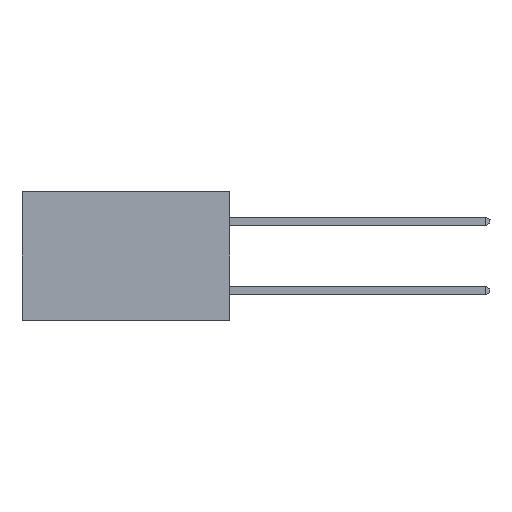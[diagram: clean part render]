
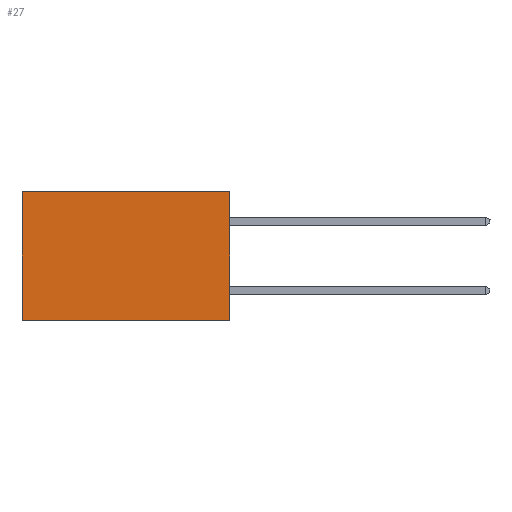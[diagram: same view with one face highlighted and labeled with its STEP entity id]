
A CAD part, left-side view. The second image highlights one B-rep face of the part: STEP entity #27.
In plain terms, the highlighted planar face has unit normal (-1, 0, 0).
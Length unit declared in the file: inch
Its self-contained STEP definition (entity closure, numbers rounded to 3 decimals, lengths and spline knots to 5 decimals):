
#27 = ADVANCED_FACE ( 'NONE', ( #2686 ), #23878, .F. ) ;
#100 = VECTOR ( 'NONE', #18522, 39.37008 ) ;
#650 = CARTESIAN_POINT ( 'NONE',  ( 0.298, 0.6, -0.37 ) ) ;
#1369 = LINE ( 'NONE', #11247, #26926 ) ;
#1914 = CARTESIAN_POINT ( 'NONE',  ( 0.298, 0.6, 0. ) ) ;
#2084 = LINE ( 'NONE', #24948, #100 ) ;
#2681 = CARTESIAN_POINT ( 'NONE',  ( 0.298, 0., 0. ) ) ;
#2686 = FACE_OUTER_BOUND ( 'NONE', #17113, .T. ) ;
#2839 = DIRECTION ( 'NONE',  ( 0., 0., -1. ) ) ;
#3073 = AXIS2_PLACEMENT_3D ( 'NONE', #2681, #17654, #5064 ) ;
#3188 = ORIENTED_EDGE ( 'NONE', *, *, #8913, .T. ) ;
#4081 = CARTESIAN_POINT ( 'NONE',  ( 0.298, 0., 0. ) ) ;
#4966 = ORIENTED_EDGE ( 'NONE', *, *, #25215, .F. ) ;
#5064 = DIRECTION ( 'NONE',  ( 0., 0., -1. ) ) ;
#8871 = VERTEX_POINT ( 'NONE', #17053 ) ;
#8913 = EDGE_CURVE ( 'NONE', #12993, #17207, #2084, .T. ) ;
#10170 = ORIENTED_EDGE ( 'NONE', *, *, #12397, .T. ) ;
#11247 = CARTESIAN_POINT ( 'NONE',  ( 0.298, 0., 0. ) ) ;
#12397 = EDGE_CURVE ( 'NONE', #17207, #14229, #22461, .T. ) ;
#12589 = VECTOR ( 'NONE', #2839, 39.37008 ) ;
#12993 = VERTEX_POINT ( 'NONE', #4081 ) ;
#13536 = CARTESIAN_POINT ( 'NONE',  ( 0.298, 0., -0.37 ) ) ;
#14229 = VERTEX_POINT ( 'NONE', #650 ) ;
#17053 = CARTESIAN_POINT ( 'NONE',  ( 0.298, 0., -0.37 ) ) ;
#17113 = EDGE_LOOP ( 'NONE', ( #10170, #17437, #4966, #3188 ) ) ;
#17207 = VERTEX_POINT ( 'NONE', #1914 ) ;
#17437 = ORIENTED_EDGE ( 'NONE', *, *, #24869, .F. ) ;
#17654 = DIRECTION ( 'NONE',  ( 1., 0., 0. ) ) ;
#17980 = DIRECTION ( 'NONE',  ( 0., 1., 0. ) ) ;
#18522 = DIRECTION ( 'NONE',  ( 0., 1., 0. ) ) ;
#20667 = LINE ( 'NONE', #13536, #23346 ) ;
#21416 = CARTESIAN_POINT ( 'NONE',  ( 0.298, 0.6, 0. ) ) ;
#22461 = LINE ( 'NONE', #21416, #12589 ) ;
#23346 = VECTOR ( 'NONE', #17980, 39.37008 ) ;
#23878 = PLANE ( 'NONE',  #3073 ) ;
#24869 = EDGE_CURVE ( 'NONE', #8871, #14229, #20667, .T. ) ;
#24948 = CARTESIAN_POINT ( 'NONE',  ( 0.298, 0., 0. ) ) ;
#25215 = EDGE_CURVE ( 'NONE', #12993, #8871, #1369, .T. ) ;
#26161 = DIRECTION ( 'NONE',  ( 0., 0., -1. ) ) ;
#26926 = VECTOR ( 'NONE', #26161, 39.37008 ) ;
